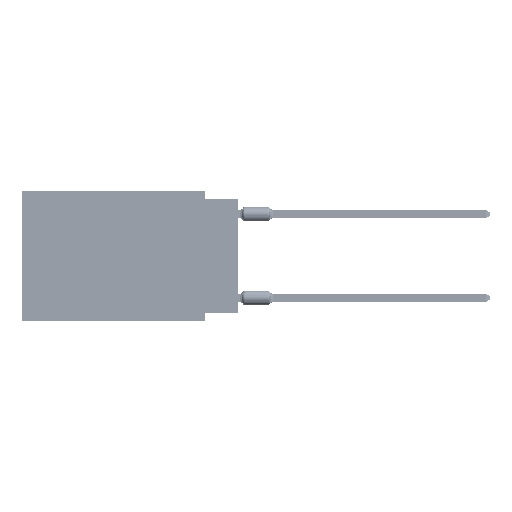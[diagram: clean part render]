
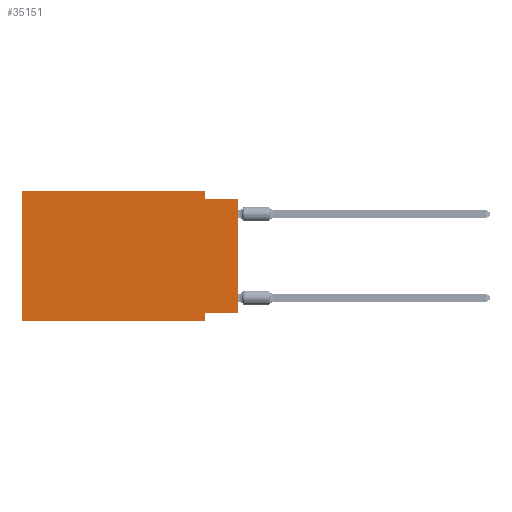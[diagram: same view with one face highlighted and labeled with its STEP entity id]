
A CAD part, left-side view. The second image highlights one B-rep face of the part: STEP entity #35151.
In plain terms, the highlighted planar face has unit normal (-1, 0, 0).
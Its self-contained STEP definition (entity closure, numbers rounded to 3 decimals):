
#4424 = EDGE_CURVE ( 'NONE', #38237, #28075, #75212, .T. ) ;
#4531 = VERTEX_POINT ( 'NONE', #70902 ) ;
#4559 = DIRECTION ( 'NONE',  ( 0., 0., -1. ) ) ;
#4836 = AXIS2_PLACEMENT_3D ( 'NONE', #82734, #55418, #4559 ) ;
#7525 = VERTEX_POINT ( 'NONE', #43294 ) ;
#8302 = VERTEX_POINT ( 'NONE', #66658 ) ;
#8789 = VECTOR ( 'NONE', #35232, 1000. ) ;
#10126 = DIRECTION ( 'NONE',  ( 0., 1., 0. ) ) ;
#10345 = VERTEX_POINT ( 'NONE', #23112 ) ;
#10432 = LINE ( 'NONE', #30099, #50129 ) ;
#17149 = LINE ( 'NONE', #29970, #32071 ) ;
#17359 = ORIENTED_EDGE ( 'NONE', *, *, #29218, .T. ) ;
#19307 = EDGE_CURVE ( 'NONE', #21356, #7525, #17149, .T. ) ;
#20627 = LINE ( 'NONE', #46269, #47946 ) ;
#21356 = VERTEX_POINT ( 'NONE', #83452 ) ;
#23112 = CARTESIAN_POINT ( 'NONE',  ( 0., 2.54, 0. ) ) ;
#24107 = VERTEX_POINT ( 'NONE', #47231 ) ;
#24154 = ORIENTED_EDGE ( 'NONE', *, *, #19307, .T. ) ;
#24932 = EDGE_CURVE ( 'NONE', #10345, #4531, #10432, .T. ) ;
#28075 = VERTEX_POINT ( 'NONE', #34686 ) ;
#29218 = EDGE_CURVE ( 'NONE', #8302, #28075, #79549, .T. ) ;
#29516 = CARTESIAN_POINT ( 'NONE',  ( 0., 2.54, -9.906 ) ) ;
#29970 = CARTESIAN_POINT ( 'NONE',  ( 0., 0., 0. ) ) ;
#30099 = CARTESIAN_POINT ( 'NONE',  ( 0., 2.54, 0. ) ) ;
#31053 = LINE ( 'NONE', #44312, #42232 ) ;
#32071 = VECTOR ( 'NONE', #55181, 1000. ) ;
#32598 = DIRECTION ( 'NONE',  ( 0., -1., 0. ) ) ;
#34104 = ORIENTED_EDGE ( 'NONE', *, *, #58635, .F. ) ;
#34686 = CARTESIAN_POINT ( 'NONE',  ( 0., 2.54, -9.906 ) ) ;
#34817 = LINE ( 'NONE', #41659, #8789 ) ;
#34934 = ORIENTED_EDGE ( 'NONE', *, *, #42421, .F. ) ;
#35151 = ADVANCED_FACE ( 'NONE', ( #81049 ), #62659, .F. ) ;
#35232 = DIRECTION ( 'NONE',  ( 0., 0., 1. ) ) ;
#35542 = ORIENTED_EDGE ( 'NONE', *, *, #4424, .F. ) ;
#37535 = VECTOR ( 'NONE', #40388, 1000. ) ;
#38237 = VERTEX_POINT ( 'NONE', #44810 ) ;
#39721 = EDGE_CURVE ( 'NONE', #21356, #38237, #31053, .T. ) ;
#40388 = DIRECTION ( 'NONE',  ( 0., -1., 0. ) ) ;
#41659 = CARTESIAN_POINT ( 'NONE',  ( 0., 16.383, 0. ) ) ;
#42232 = VECTOR ( 'NONE', #10126, 1000. ) ;
#42421 = EDGE_CURVE ( 'NONE', #4531, #7525, #20627, .T. ) ;
#43294 = CARTESIAN_POINT ( 'NONE',  ( 0., 0., -0.635 ) ) ;
#44312 = CARTESIAN_POINT ( 'NONE',  ( 0., 0., -9.271 ) ) ;
#44355 = ORIENTED_EDGE ( 'NONE', *, *, #24932, .F. ) ;
#44798 = ORIENTED_EDGE ( 'NONE', *, *, #39721, .F. ) ;
#44810 = CARTESIAN_POINT ( 'NONE',  ( 0., 2.54, -9.271 ) ) ;
#45838 = CARTESIAN_POINT ( 'NONE',  ( 0., 16.383, -9.906 ) ) ;
#46269 = CARTESIAN_POINT ( 'NONE',  ( 0., 0., -0.635 ) ) ;
#47231 = CARTESIAN_POINT ( 'NONE',  ( 0., 16.383, 0. ) ) ;
#47946 = VECTOR ( 'NONE', #32598, 1000. ) ;
#50129 = VECTOR ( 'NONE', #83888, 1000. ) ;
#53178 = LINE ( 'NONE', #72811, #37535 ) ;
#55181 = DIRECTION ( 'NONE',  ( 0., 0., 1. ) ) ;
#55418 = DIRECTION ( 'NONE',  ( 1., 0., 0. ) ) ;
#58635 = EDGE_CURVE ( 'NONE', #24107, #10345, #53178, .T. ) ;
#59222 = EDGE_LOOP ( 'NONE', ( #24154, #34934, #44355, #34104, #66812, #17359, #35542, #44798 ) ) ;
#59817 = EDGE_CURVE ( 'NONE', #8302, #24107, #34817, .T. ) ;
#62659 = PLANE ( 'NONE',  #4836 ) ;
#63695 = VECTOR ( 'NONE', #81618, 1000. ) ;
#66658 = CARTESIAN_POINT ( 'NONE',  ( 0., 16.383, -9.906 ) ) ;
#66812 = ORIENTED_EDGE ( 'NONE', *, *, #59817, .F. ) ;
#70902 = CARTESIAN_POINT ( 'NONE',  ( 0., 2.54, -0.635 ) ) ;
#72811 = CARTESIAN_POINT ( 'NONE',  ( 0., 16.383, 0. ) ) ;
#73566 = VECTOR ( 'NONE', #78705, 1000. ) ;
#75212 = LINE ( 'NONE', #29516, #63695 ) ;
#78705 = DIRECTION ( 'NONE',  ( 0., -1., 0. ) ) ;
#79549 = LINE ( 'NONE', #45838, #73566 ) ;
#81049 = FACE_OUTER_BOUND ( 'NONE', #59222, .T. ) ;
#81618 = DIRECTION ( 'NONE',  ( 0., 0., -1. ) ) ;
#82734 = CARTESIAN_POINT ( 'NONE',  ( 0., 16.383, 0. ) ) ;
#83452 = CARTESIAN_POINT ( 'NONE',  ( 0., 0., -9.271 ) ) ;
#83888 = DIRECTION ( 'NONE',  ( 0., 0., -1. ) ) ;
